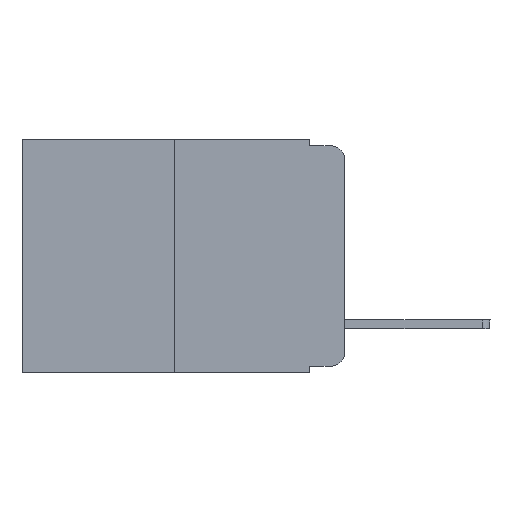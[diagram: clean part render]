
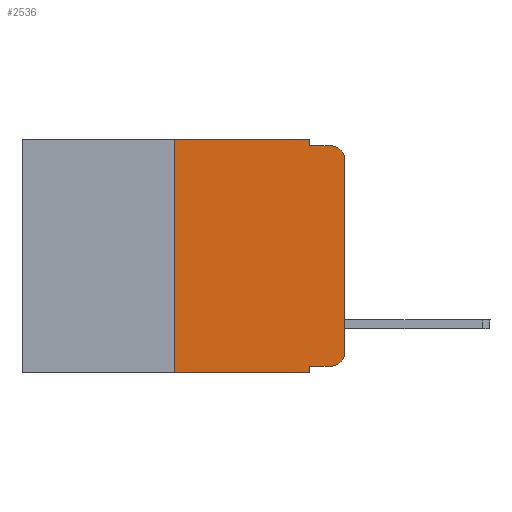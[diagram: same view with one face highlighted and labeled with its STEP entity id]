
A CAD part, left-side view. The second image highlights one B-rep face of the part: STEP entity #2536.
In plain terms, the highlighted planar face has unit normal (-1, 0, 0).
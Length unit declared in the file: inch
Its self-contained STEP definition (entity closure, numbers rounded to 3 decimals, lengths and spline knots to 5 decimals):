
#31 = VERTEX_POINT ( 'NONE', #10441 ) ;
#250 = DIRECTION ( 'NONE',  ( -1., 0., 0. ) ) ;
#270 = CARTESIAN_POINT ( 'NONE',  ( 0., 0.051, -0.333 ) ) ;
#1108 = CARTESIAN_POINT ( 'NONE',  ( 0., 0.25, 0. ) ) ;
#1196 = VECTOR ( 'NONE', #1212, 39.37008 ) ;
#1212 = DIRECTION ( 'NONE',  ( 0., -1., 0. ) ) ;
#1328 = VERTEX_POINT ( 'NONE', #4362 ) ;
#1495 = AXIS2_PLACEMENT_3D ( 'NONE', #3400, #11339, #11225 ) ;
#1530 = VERTEX_POINT ( 'NONE', #11090 ) ;
#1686 = CARTESIAN_POINT ( 'NONE',  ( 0., 0.25, 0. ) ) ;
#1721 = ORIENTED_EDGE ( 'NONE', *, *, #4703, .F. ) ;
#1932 = DIRECTION ( 'NONE',  ( 0., 0., -1. ) ) ;
#1990 = ORIENTED_EDGE ( 'NONE', *, *, #3288, .T. ) ;
#2023 = CARTESIAN_POINT ( 'NONE',  ( 0., 0.051, 0. ) ) ;
#2066 = CARTESIAN_POINT ( 'NONE',  ( 0., 0.473, 0. ) ) ;
#2536 = ADVANCED_FACE ( 'NONE', ( #4683 ), #7439, .F. ) ;
#2776 = ORIENTED_EDGE ( 'NONE', *, *, #3530, .F. ) ;
#2793 = VERTEX_POINT ( 'NONE', #8743 ) ;
#2848 = ORIENTED_EDGE ( 'NONE', *, *, #10662, .F. ) ;
#3075 = CARTESIAN_POINT ( 'NONE',  ( 0., 0.473, 0. ) ) ;
#3288 = EDGE_CURVE ( 'NONE', #6663, #31, #7929, .T. ) ;
#3349 = DIRECTION ( 'NONE',  ( 0., 0., 1. ) ) ;
#3400 = CARTESIAN_POINT ( 'NONE',  ( 0., 0.02, -0.313 ) ) ;
#3417 = CIRCLE ( 'NONE', #1495, 0.02 ) ;
#3513 = CARTESIAN_POINT ( 'NONE',  ( 0., 0.051, 0. ) ) ;
#3530 = EDGE_CURVE ( 'NONE', #10666, #8390, #8628, .T. ) ;
#3546 = EDGE_CURVE ( 'NONE', #1328, #8390, #4521, .T. ) ;
#3594 = ORIENTED_EDGE ( 'NONE', *, *, #3636, .T. ) ;
#3605 = DIRECTION ( 'NONE',  ( 0., 0., -1. ) ) ;
#3636 = EDGE_CURVE ( 'NONE', #10666, #2793, #8048, .T. ) ;
#3701 = CARTESIAN_POINT ( 'NONE',  ( 0., 0.051, -0.343 ) ) ;
#3800 = CARTESIAN_POINT ( 'NONE',  ( 0., 0.051, -0.333 ) ) ;
#3938 = DIRECTION ( 'NONE',  ( 0., -1., 0. ) ) ;
#4084 = AXIS2_PLACEMENT_3D ( 'NONE', #3075, #8397, #4897 ) ;
#4259 = LINE ( 'NONE', #1108, #7511 ) ;
#4362 = CARTESIAN_POINT ( 'NONE',  ( 0., 0.25, -0.343 ) ) ;
#4386 = VECTOR ( 'NONE', #5660, 39.37008 ) ;
#4391 = VECTOR ( 'NONE', #8937, 39.37008 ) ;
#4482 = EDGE_CURVE ( 'NONE', #2793, #6663, #3417, .T. ) ;
#4511 = VERTEX_POINT ( 'NONE', #1686 ) ;
#4521 = LINE ( 'NONE', #10766, #4386 ) ;
#4526 = LINE ( 'NONE', #7881, #4391 ) ;
#4683 = FACE_OUTER_BOUND ( 'NONE', #5616, .T. ) ;
#4703 = EDGE_CURVE ( 'NONE', #1328, #4511, #4259, .T. ) ;
#4897 = DIRECTION ( 'NONE',  ( 0., 0., -1. ) ) ;
#4906 = LINE ( 'NONE', #2066, #11107 ) ;
#4967 = LINE ( 'NONE', #2023, #11441 ) ;
#5360 = CARTESIAN_POINT ( 'NONE',  ( 0., 0.051, 0. ) ) ;
#5562 = CARTESIAN_POINT ( 'NONE',  ( 0., 0.02, -0.03 ) ) ;
#5616 = EDGE_LOOP ( 'NONE', ( #1990, #10921, #9417, #2848, #8476, #1721, #5836, #2776, #3594, #11174 ) ) ;
#5660 = DIRECTION ( 'NONE',  ( 0., -1., 0. ) ) ;
#5836 = ORIENTED_EDGE ( 'NONE', *, *, #3546, .T. ) ;
#6419 = DIRECTION ( 'NONE',  ( 0., 0., -1. ) ) ;
#6663 = VERTEX_POINT ( 'NONE', #8600 ) ;
#6823 = CIRCLE ( 'NONE', #10489, 0.02 ) ;
#7247 = DIRECTION ( 'NONE',  ( 0., 0., 1. ) ) ;
#7385 = VECTOR ( 'NONE', #3605, 39.37008 ) ;
#7439 = PLANE ( 'NONE',  #4084 ) ;
#7511 = VECTOR ( 'NONE', #7247, 39.37008 ) ;
#7630 = CARTESIAN_POINT ( 'NONE',  ( 0., 0.051, -0.01 ) ) ;
#7881 = CARTESIAN_POINT ( 'NONE',  ( 0., 0.051, -0.01 ) ) ;
#7929 = LINE ( 'NONE', #9473, #9352 ) ;
#8048 = LINE ( 'NONE', #270, #1196 ) ;
#8390 = VERTEX_POINT ( 'NONE', #3701 ) ;
#8397 = DIRECTION ( 'NONE',  ( 1., 0., 0. ) ) ;
#8476 = ORIENTED_EDGE ( 'NONE', *, *, #8626, .F. ) ;
#8600 = CARTESIAN_POINT ( 'NONE',  ( 0., 0., -0.313 ) ) ;
#8620 = EDGE_CURVE ( 'NONE', #31, #1530, #6823, .T. ) ;
#8626 = EDGE_CURVE ( 'NONE', #4511, #9824, #4906, .T. ) ;
#8628 = LINE ( 'NONE', #5360, #7385 ) ;
#8743 = CARTESIAN_POINT ( 'NONE',  ( 0., 0.02, -0.333 ) ) ;
#8937 = DIRECTION ( 'NONE',  ( 0., -1., 0. ) ) ;
#9352 = VECTOR ( 'NONE', #3349, 39.37008 ) ;
#9417 = ORIENTED_EDGE ( 'NONE', *, *, #11244, .F. ) ;
#9473 = CARTESIAN_POINT ( 'NONE',  ( 0., 0., 0. ) ) ;
#9824 = VERTEX_POINT ( 'NONE', #3513 ) ;
#10441 = CARTESIAN_POINT ( 'NONE',  ( 0., 0., -0.03 ) ) ;
#10489 = AXIS2_PLACEMENT_3D ( 'NONE', #5562, #250, #6419 ) ;
#10662 = EDGE_CURVE ( 'NONE', #9824, #10967, #4967, .T. ) ;
#10666 = VERTEX_POINT ( 'NONE', #3800 ) ;
#10766 = CARTESIAN_POINT ( 'NONE',  ( 0., 0.473, -0.343 ) ) ;
#10921 = ORIENTED_EDGE ( 'NONE', *, *, #8620, .T. ) ;
#10967 = VERTEX_POINT ( 'NONE', #7630 ) ;
#11090 = CARTESIAN_POINT ( 'NONE',  ( 0., 0.02, -0.01 ) ) ;
#11107 = VECTOR ( 'NONE', #3938, 39.37008 ) ;
#11174 = ORIENTED_EDGE ( 'NONE', *, *, #4482, .T. ) ;
#11225 = DIRECTION ( 'NONE',  ( 0., 0., -1. ) ) ;
#11244 = EDGE_CURVE ( 'NONE', #10967, #1530, #4526, .T. ) ;
#11339 = DIRECTION ( 'NONE',  ( -1., 0., 0. ) ) ;
#11441 = VECTOR ( 'NONE', #1932, 39.37008 ) ;
